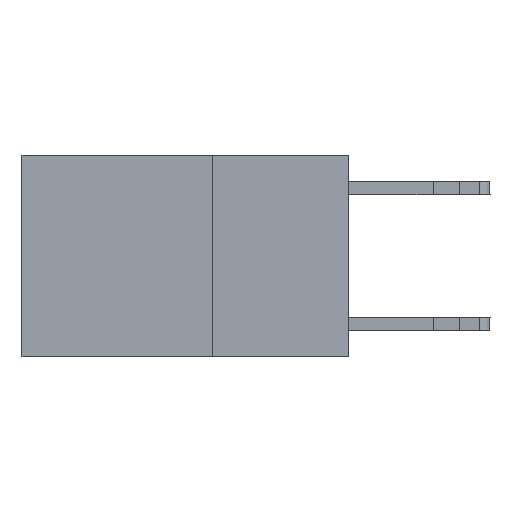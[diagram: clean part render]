
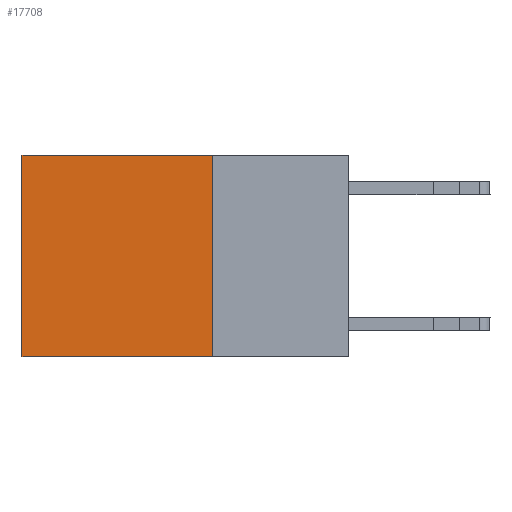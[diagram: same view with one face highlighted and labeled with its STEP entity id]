
A CAD part, left-side view. The second image highlights one B-rep face of the part: STEP entity #17708.
In plain terms, the highlighted planar face has unit normal (-1, 0, 0).
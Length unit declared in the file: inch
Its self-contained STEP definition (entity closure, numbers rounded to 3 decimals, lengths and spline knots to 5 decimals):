
#66 = CARTESIAN_POINT ( 'NONE',  ( 0.2625, 0.6, 0. ) ) ;
#323 = LINE ( 'NONE', #13812, #17774 ) ;
#1726 = CARTESIAN_POINT ( 'NONE',  ( 0.2625, 0.25, -0.37 ) ) ;
#1857 = EDGE_CURVE ( 'NONE', #4268, #21130, #18297, .T. ) ;
#1953 = EDGE_CURVE ( 'NONE', #7755, #4268, #10574, .T. ) ;
#3261 = DIRECTION ( 'NONE',  ( 0., 1., 0. ) ) ;
#4268 = VERTEX_POINT ( 'NONE', #17198 ) ;
#5138 = DIRECTION ( 'NONE',  ( 1., 0., 0. ) ) ;
#5669 = ORIENTED_EDGE ( 'NONE', *, *, #1857, .F. ) ;
#7126 = CARTESIAN_POINT ( 'NONE',  ( 0.2625, 0.25, 0. ) ) ;
#7755 = VERTEX_POINT ( 'NONE', #7126 ) ;
#8223 = EDGE_CURVE ( 'NONE', #7755, #9041, #323, .T. ) ;
#8457 = FACE_OUTER_BOUND ( 'NONE', #18743, .T. ) ;
#9041 = VERTEX_POINT ( 'NONE', #66 ) ;
#10574 = LINE ( 'NONE', #20921, #20636 ) ;
#11084 = DIRECTION ( 'NONE',  ( 0., 0., -1. ) ) ;
#11450 = CARTESIAN_POINT ( 'NONE',  ( 0.2625, 0.25, 0. ) ) ;
#11556 = CARTESIAN_POINT ( 'NONE',  ( 0.2625, 0.6, -0.37 ) ) ;
#11773 = DIRECTION ( 'NONE',  ( 0., 0., -1. ) ) ;
#11787 = VECTOR ( 'NONE', #11084, 39.37008 ) ;
#11832 = VECTOR ( 'NONE', #3261, 39.37008 ) ;
#12615 = LINE ( 'NONE', #12718, #11787 ) ;
#12718 = CARTESIAN_POINT ( 'NONE',  ( 0.2625, 0.6, 0. ) ) ;
#12934 = EDGE_CURVE ( 'NONE', #9041, #21130, #12615, .T. ) ;
#13812 = CARTESIAN_POINT ( 'NONE',  ( 0.2625, 0.25, 0. ) ) ;
#14969 = PLANE ( 'NONE',  #20673 ) ;
#15848 = DIRECTION ( 'NONE',  ( 0., 0., -1. ) ) ;
#17198 = CARTESIAN_POINT ( 'NONE',  ( 0.2625, 0.25, -0.37 ) ) ;
#17233 = DIRECTION ( 'NONE',  ( 0., 1., 0. ) ) ;
#17708 = ADVANCED_FACE ( 'NONE', ( #8457 ), #14969, .F. ) ;
#17774 = VECTOR ( 'NONE', #17233, 39.37008 ) ;
#18297 = LINE ( 'NONE', #1726, #11832 ) ;
#18670 = ORIENTED_EDGE ( 'NONE', *, *, #12934, .T. ) ;
#18743 = EDGE_LOOP ( 'NONE', ( #18670, #5669, #19050, #18924 ) ) ;
#18924 = ORIENTED_EDGE ( 'NONE', *, *, #8223, .T. ) ;
#19050 = ORIENTED_EDGE ( 'NONE', *, *, #1953, .F. ) ;
#20636 = VECTOR ( 'NONE', #15848, 39.37008 ) ;
#20673 = AXIS2_PLACEMENT_3D ( 'NONE', #11450, #5138, #11773 ) ;
#20921 = CARTESIAN_POINT ( 'NONE',  ( 0.2625, 0.25, 0. ) ) ;
#21130 = VERTEX_POINT ( 'NONE', #11556 ) ;
